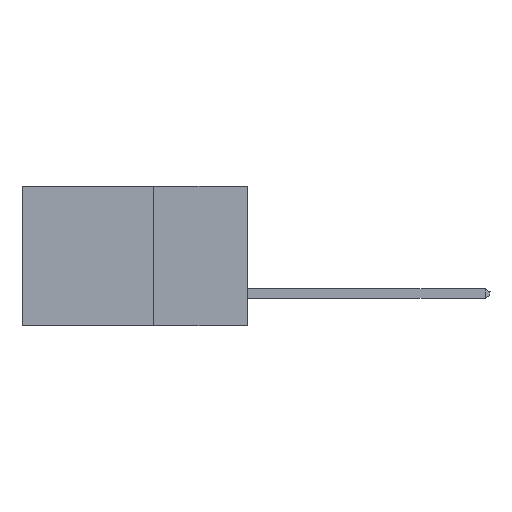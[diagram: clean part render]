
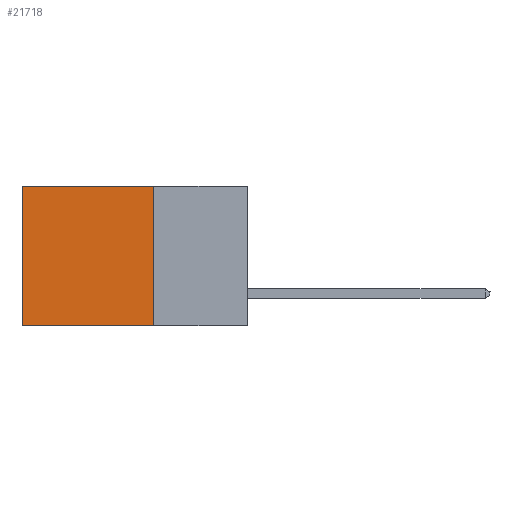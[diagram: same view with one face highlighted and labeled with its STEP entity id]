
A CAD part, left-side view. The second image highlights one B-rep face of the part: STEP entity #21718.
In plain terms, the highlighted planar face has unit normal (-1, 0, 0).
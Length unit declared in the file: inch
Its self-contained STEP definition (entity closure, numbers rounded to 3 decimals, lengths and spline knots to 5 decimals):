
#300 = CARTESIAN_POINT ( 'NONE',  ( 0.2615, 0.6, -0.37 ) ) ;
#1257 = EDGE_CURVE ( 'NONE', #4711, #17313, #4629, .T. ) ;
#2142 = ORIENTED_EDGE ( 'NONE', *, *, #19476, .T. ) ;
#2293 = ORIENTED_EDGE ( 'NONE', *, *, #14777, .T. ) ;
#2527 = ORIENTED_EDGE ( 'NONE', *, *, #1257, .F. ) ;
#4629 = LINE ( 'NONE', #6288, #17739 ) ;
#4711 = VERTEX_POINT ( 'NONE', #15630 ) ;
#4999 = VECTOR ( 'NONE', #13656, 39.37008 ) ;
#6022 = CARTESIAN_POINT ( 'NONE',  ( 0.2615, 0.25, 0. ) ) ;
#6288 = CARTESIAN_POINT ( 'NONE',  ( 0.2615, 0.25, -0.37 ) ) ;
#6451 = CARTESIAN_POINT ( 'NONE',  ( 0.2615, 0.6, -0.37 ) ) ;
#8236 = LINE ( 'NONE', #6451, #4999 ) ;
#8798 = PLANE ( 'NONE',  #17159 ) ;
#9928 = DIRECTION ( 'NONE',  ( 0., 1., 0. ) ) ;
#10518 = VECTOR ( 'NONE', #9928, 39.37008 ) ;
#12351 = VERTEX_POINT ( 'NONE', #15124 ) ;
#12409 = EDGE_CURVE ( 'NONE', #17313, #23515, #13586, .T. ) ;
#13468 = CARTESIAN_POINT ( 'NONE',  ( 0.2615, 0.25, -0.37 ) ) ;
#13586 = LINE ( 'NONE', #13468, #10518 ) ;
#13656 = DIRECTION ( 'NONE',  ( 0., 0., -1. ) ) ;
#14123 = DIRECTION ( 'NONE',  ( 1., 0., 0. ) ) ;
#14777 = EDGE_CURVE ( 'NONE', #12351, #23515, #8236, .T. ) ;
#15124 = CARTESIAN_POINT ( 'NONE',  ( 0.2615, 0.6, 0. ) ) ;
#15630 = CARTESIAN_POINT ( 'NONE',  ( 0.2615, 0.25, 0. ) ) ;
#16906 = DIRECTION ( 'NONE',  ( 0., 1., 0. ) ) ;
#16947 = CARTESIAN_POINT ( 'NONE',  ( 0.2615, 0.25, -0.37 ) ) ;
#17159 = AXIS2_PLACEMENT_3D ( 'NONE', #17667, #14123, #23425 ) ;
#17288 = DIRECTION ( 'NONE',  ( 0., 0., -1. ) ) ;
#17313 = VERTEX_POINT ( 'NONE', #16947 ) ;
#17667 = CARTESIAN_POINT ( 'NONE',  ( 0.2615, 0.25, -0.37 ) ) ;
#17739 = VECTOR ( 'NONE', #17288, 39.37008 ) ;
#18717 = EDGE_LOOP ( 'NONE', ( #2293, #20131, #2527, #2142 ) ) ;
#19476 = EDGE_CURVE ( 'NONE', #4711, #12351, #22174, .T. ) ;
#20131 = ORIENTED_EDGE ( 'NONE', *, *, #12409, .F. ) ;
#21621 = FACE_OUTER_BOUND ( 'NONE', #18717, .T. ) ;
#21718 = ADVANCED_FACE ( 'NONE', ( #21621 ), #8798, .F. ) ;
#22174 = LINE ( 'NONE', #6022, #22429 ) ;
#22429 = VECTOR ( 'NONE', #16906, 39.37008 ) ;
#23425 = DIRECTION ( 'NONE',  ( 0., 0., -1. ) ) ;
#23515 = VERTEX_POINT ( 'NONE', #300 ) ;
